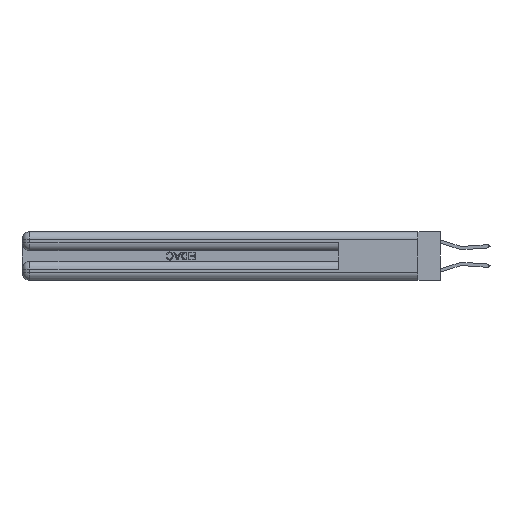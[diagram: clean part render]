
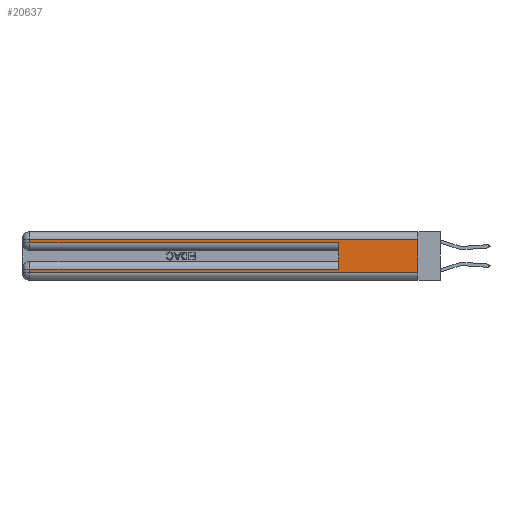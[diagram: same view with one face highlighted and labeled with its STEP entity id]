
A CAD part, left-side view. The second image highlights one B-rep face of the part: STEP entity #20637.
In plain terms, the highlighted planar face has unit normal (-1, 0, 0).
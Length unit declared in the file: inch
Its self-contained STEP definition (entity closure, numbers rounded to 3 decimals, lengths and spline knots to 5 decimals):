
#110 = VECTOR ( 'NONE', #16410, 39.37008 ) ;
#154 = EDGE_CURVE ( 'NONE', #7273, #20300, #29478, .T. ) ;
#315 = FACE_OUTER_BOUND ( 'NONE', #3330, .T. ) ;
#1510 = ORIENTED_EDGE ( 'NONE', *, *, #22359, .T. ) ;
#2243 = LINE ( 'NONE', #32302, #31340 ) ;
#2698 = LINE ( 'NONE', #13602, #9792 ) ;
#2883 = DIRECTION ( 'NONE',  ( 0., 0., -1. ) ) ;
#3140 = LINE ( 'NONE', #3319, #33258 ) ;
#3171 = PLANE ( 'NONE',  #9509 ) ;
#3319 = CARTESIAN_POINT ( 'NONE',  ( 0., 0., 0.285 ) ) ;
#3330 = EDGE_LOOP ( 'NONE', ( #31438, #5458, #18855, #14006, #12737, #12767, #1510, #15350 ) ) ;
#3351 = VERTEX_POINT ( 'NONE', #8354 ) ;
#3841 = DIRECTION ( 'NONE',  ( 0., 0., -1. ) ) ;
#4433 = CARTESIAN_POINT ( 'NONE',  ( 0., 0., 0.06 ) ) ;
#5065 = EDGE_CURVE ( 'NONE', #13490, #6538, #2243, .T. ) ;
#5458 = ORIENTED_EDGE ( 'NONE', *, *, #18719, .T. ) ;
#5494 = CARTESIAN_POINT ( 'NONE',  ( 0., 0.6, 0.145 ) ) ;
#6538 = VERTEX_POINT ( 'NONE', #4433 ) ;
#7124 = VECTOR ( 'NONE', #25584, 39.37008 ) ;
#7273 = VERTEX_POINT ( 'NONE', #9353 ) ;
#8354 = CARTESIAN_POINT ( 'NONE',  ( 0., 2.94, 0.31 ) ) ;
#9353 = CARTESIAN_POINT ( 'NONE',  ( 0., 0.6, 0.085 ) ) ;
#9509 = AXIS2_PLACEMENT_3D ( 'NONE', #11225, #22135, #11758 ) ;
#9792 = VECTOR ( 'NONE', #2883, 39.37008 ) ;
#11134 = DIRECTION ( 'NONE',  ( 0., 1., 0. ) ) ;
#11225 = CARTESIAN_POINT ( 'NONE',  ( 0., 0., 0.37 ) ) ;
#11306 = VERTEX_POINT ( 'NONE', #12880 ) ;
#11725 = DIRECTION ( 'NONE',  ( 0., 0., -1. ) ) ;
#11758 = DIRECTION ( 'NONE',  ( 0., 0., -1. ) ) ;
#11948 = CARTESIAN_POINT ( 'NONE',  ( 0., 2.94, 0.06 ) ) ;
#12486 = EDGE_CURVE ( 'NONE', #11306, #6538, #32508, .T. ) ;
#12737 = ORIENTED_EDGE ( 'NONE', *, *, #154, .F. ) ;
#12767 = ORIENTED_EDGE ( 'NONE', *, *, #22763, .T. ) ;
#12880 = CARTESIAN_POINT ( 'NONE',  ( 0., 0., 0.31 ) ) ;
#12939 = EDGE_CURVE ( 'NONE', #3351, #20362, #2698, .T. ) ;
#13191 = VECTOR ( 'NONE', #11725, 39.37008 ) ;
#13490 = VERTEX_POINT ( 'NONE', #11948 ) ;
#13602 = CARTESIAN_POINT ( 'NONE',  ( 0., 2.94, 0.37 ) ) ;
#14006 = ORIENTED_EDGE ( 'NONE', *, *, #15354, .T. ) ;
#14130 = CARTESIAN_POINT ( 'NONE',  ( 0., 0., 0.31 ) ) ;
#15350 = ORIENTED_EDGE ( 'NONE', *, *, #5065, .T. ) ;
#15354 = EDGE_CURVE ( 'NONE', #20362, #20300, #3140, .T. ) ;
#16410 = DIRECTION ( 'NONE',  ( 0., 0., 1. ) ) ;
#16506 = CARTESIAN_POINT ( 'NONE',  ( 0., 0.6, 0.285 ) ) ;
#16520 = CARTESIAN_POINT ( 'NONE',  ( 0., 0., 0.085 ) ) ;
#17277 = LINE ( 'NONE', #28016, #33998 ) ;
#18570 = VECTOR ( 'NONE', #11134, 39.37008 ) ;
#18719 = EDGE_CURVE ( 'NONE', #11306, #3351, #33650, .T. ) ;
#18855 = ORIENTED_EDGE ( 'NONE', *, *, #12939, .T. ) ;
#18893 = CARTESIAN_POINT ( 'NONE',  ( 0., 0., 0.37 ) ) ;
#20300 = VERTEX_POINT ( 'NONE', #16506 ) ;
#20362 = VERTEX_POINT ( 'NONE', #26805 ) ;
#20637 = ADVANCED_FACE ( 'NONE', ( #315 ), #3171, .F. ) ;
#22052 = LINE ( 'NONE', #16520, #18570 ) ;
#22135 = DIRECTION ( 'NONE',  ( 1., 0., 0. ) ) ;
#22359 = EDGE_CURVE ( 'NONE', #27222, #13490, #17277, .T. ) ;
#22763 = EDGE_CURVE ( 'NONE', #7273, #27222, #22052, .T. ) ;
#25584 = DIRECTION ( 'NONE',  ( 0., 1., 0. ) ) ;
#26805 = CARTESIAN_POINT ( 'NONE',  ( 0., 2.94, 0.285 ) ) ;
#27222 = VERTEX_POINT ( 'NONE', #31546 ) ;
#28016 = CARTESIAN_POINT ( 'NONE',  ( 0., 2.94, 0.37 ) ) ;
#29478 = LINE ( 'NONE', #5494, #110 ) ;
#31340 = VECTOR ( 'NONE', #34625, 39.37008 ) ;
#31438 = ORIENTED_EDGE ( 'NONE', *, *, #12486, .F. ) ;
#31546 = CARTESIAN_POINT ( 'NONE',  ( 0., 2.94, 0.085 ) ) ;
#32302 = CARTESIAN_POINT ( 'NONE',  ( 0., 0., 0.06 ) ) ;
#32508 = LINE ( 'NONE', #18893, #13191 ) ;
#33258 = VECTOR ( 'NONE', #33568, 39.37008 ) ;
#33568 = DIRECTION ( 'NONE',  ( 0., -1., 0. ) ) ;
#33650 = LINE ( 'NONE', #14130, #7124 ) ;
#33998 = VECTOR ( 'NONE', #3841, 39.37008 ) ;
#34625 = DIRECTION ( 'NONE',  ( 0., -1., 0. ) ) ;
